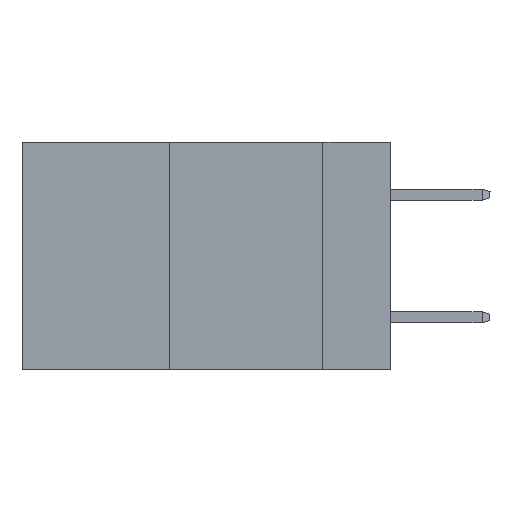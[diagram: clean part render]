
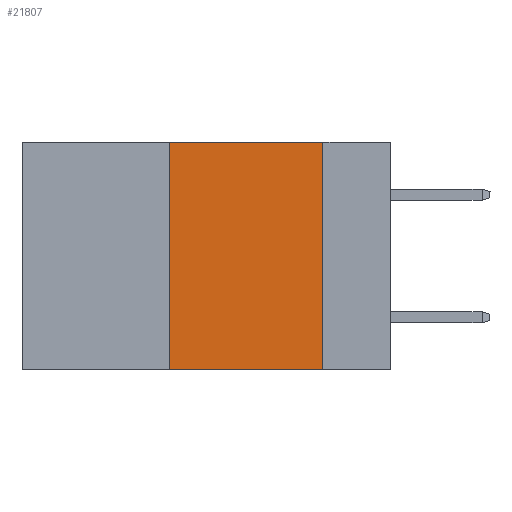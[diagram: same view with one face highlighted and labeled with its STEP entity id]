
A CAD part, left-side view. The second image highlights one B-rep face of the part: STEP entity #21807.
In plain terms, the highlighted planar face has unit normal (-1, 0, 0).
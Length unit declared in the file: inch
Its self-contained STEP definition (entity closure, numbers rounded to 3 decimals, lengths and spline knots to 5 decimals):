
#271 = VECTOR ( 'NONE', #36702, 39.37008 ) ;
#1161 = CARTESIAN_POINT ( 'NONE',  ( 0., 0.11, 0. ) ) ;
#1589 = LINE ( 'NONE', #1161, #10390 ) ;
#2844 = CARTESIAN_POINT ( 'NONE',  ( 0., 0.36, -0.37 ) ) ;
#3200 = VECTOR ( 'NONE', #7947, 39.37008 ) ;
#6221 = EDGE_CURVE ( 'NONE', #41736, #34304, #33417, .T. ) ;
#6836 = CARTESIAN_POINT ( 'NONE',  ( 0., 0.6, 0. ) ) ;
#7947 = DIRECTION ( 'NONE',  ( 0., -1., 0. ) ) ;
#8419 = LINE ( 'NONE', #35439, #13180 ) ;
#10390 = VECTOR ( 'NONE', #20934, 39.37008 ) ;
#10569 = DIRECTION ( 'NONE',  ( 0., 0., -1. ) ) ;
#10902 = ORIENTED_EDGE ( 'NONE', *, *, #6221, .F. ) ;
#11468 = CARTESIAN_POINT ( 'NONE',  ( 0., 0.6, -0.37 ) ) ;
#13180 = VECTOR ( 'NONE', #32568, 39.37008 ) ;
#14011 = EDGE_CURVE ( 'NONE', #14665, #41736, #8419, .T. ) ;
#14665 = VERTEX_POINT ( 'NONE', #2844 ) ;
#18279 = LINE ( 'NONE', #11468, #3200 ) ;
#19141 = CARTESIAN_POINT ( 'NONE',  ( 0., 0.6, 0. ) ) ;
#20229 = FACE_OUTER_BOUND ( 'NONE', #21315, .T. ) ;
#20251 = EDGE_CURVE ( 'NONE', #34304, #25065, #1589, .T. ) ;
#20882 = DIRECTION ( 'NONE',  ( 1., 0., 0. ) ) ;
#20934 = DIRECTION ( 'NONE',  ( 0., 0., -1. ) ) ;
#21315 = EDGE_LOOP ( 'NONE', ( #41570, #10902, #30090, #39886 ) ) ;
#21807 = ADVANCED_FACE ( 'NONE', ( #20229 ), #27486, .F. ) ;
#23804 = AXIS2_PLACEMENT_3D ( 'NONE', #6836, #20882, #10569 ) ;
#24868 = CARTESIAN_POINT ( 'NONE',  ( 0., 0.11, 0. ) ) ;
#25065 = VERTEX_POINT ( 'NONE', #43054 ) ;
#27486 = PLANE ( 'NONE',  #23804 ) ;
#30090 = ORIENTED_EDGE ( 'NONE', *, *, #14011, .F. ) ;
#31359 = CARTESIAN_POINT ( 'NONE',  ( 0., 0.36, 0. ) ) ;
#32568 = DIRECTION ( 'NONE',  ( 0., 0., 1. ) ) ;
#33417 = LINE ( 'NONE', #19141, #271 ) ;
#34297 = EDGE_CURVE ( 'NONE', #14665, #25065, #18279, .T. ) ;
#34304 = VERTEX_POINT ( 'NONE', #24868 ) ;
#35439 = CARTESIAN_POINT ( 'NONE',  ( 0., 0.36, 0. ) ) ;
#36702 = DIRECTION ( 'NONE',  ( 0., -1., 0. ) ) ;
#39886 = ORIENTED_EDGE ( 'NONE', *, *, #34297, .T. ) ;
#41570 = ORIENTED_EDGE ( 'NONE', *, *, #20251, .F. ) ;
#41736 = VERTEX_POINT ( 'NONE', #31359 ) ;
#43054 = CARTESIAN_POINT ( 'NONE',  ( 0., 0.11, -0.37 ) ) ;
